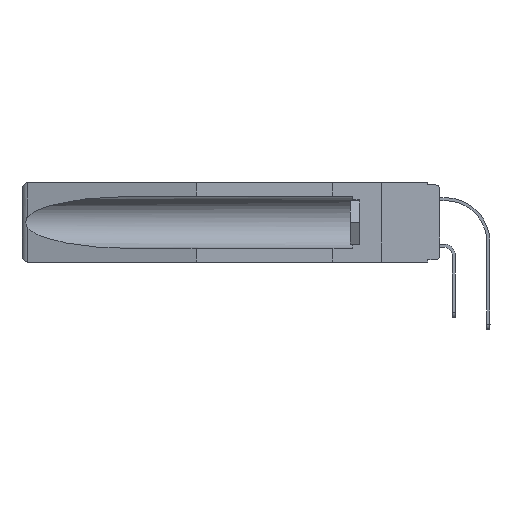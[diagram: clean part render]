
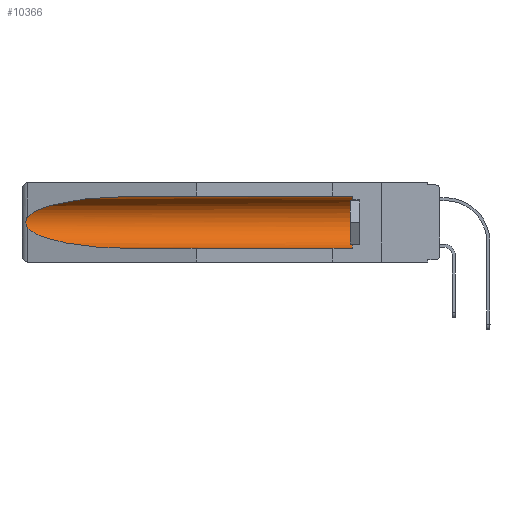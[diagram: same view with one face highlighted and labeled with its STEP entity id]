
A CAD part, left-side view. The second image highlights one B-rep face of the part: STEP entity #10366.
In plain terms, the highlighted cylindrical face has radius 2.857 mm (diameter 5.715 mm), a partial arc.
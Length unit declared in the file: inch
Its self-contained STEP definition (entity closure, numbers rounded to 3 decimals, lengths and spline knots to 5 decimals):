
#819 = VECTOR ( 'NONE', #11429, 39.37008 ) ;
#1091 = EDGE_CURVE ( 'NONE', #2972, #17838, #14023, .T. ) ;
#1241 = ORIENTED_EDGE ( 'NONE', *, *, #8715, .F. ) ;
#1884 = VECTOR ( 'NONE', #8492, 39.37008 ) ;
#2430 = CARTESIAN_POINT ( 'NONE',  ( 0.155, 1.07973, -0.284 ) ) ;
#2876 = CARTESIAN_POINT ( 'NONE',  ( 0.26597, 1.5296, -0.19026 ) ) ;
#2972 = VERTEX_POINT ( 'NONE', #4552 ) ;
#3889 = CYLINDRICAL_SURFACE ( 'NONE', #4646, 0.1125 ) ;
#4006 = CARTESIAN_POINT ( 'NONE',  ( 0.2675, 1.53308, -0.16763 ) ) ;
#4163 = CARTESIAN_POINT ( 'NONE',  ( 0.155, 1.07973, -0.059 ) ) ;
#4523 = EDGE_LOOP ( 'NONE', ( #17847, #11388, #7519, #1241, #16704, #6008 ) ) ;
#4552 = CARTESIAN_POINT ( 'NONE',  ( 0.155, 0.126, -0.059 ) ) ;
#4646 = AXIS2_PLACEMENT_3D ( 'NONE', #16730, #8152, #13783 ) ;
#4809 =( BOUNDED_CURVE ( )  B_SPLINE_CURVE ( 3, ( #4163, #5647, #17003, #9745 ),
 .UNSPECIFIED., .F., .F. ) 
 B_SPLINE_CURVE_WITH_KNOTS ( ( 4, 4 ),
 ( 4.71239, 6.08839 ),
 .UNSPECIFIED. ) 
 CURVE ( )  GEOMETRIC_REPRESENTATION_ITEM ( )  RATIONAL_B_SPLINE_CURVE ( ( 1., 0.848, 0.848, 1. ) ) 
 REPRESENTATION_ITEM ( '' )  );
#5072 = B_SPLINE_CURVE_WITH_KNOTS ( 'NONE', 3,
 ( #14075, #11043, #15450, #5665, #4006, #6882, #12518, #9936, #2876, #8532 ),
 .UNSPECIFIED., .F., .F.,
 ( 4, 2, 2, 2, 4 ),
 ( 0., 0.00029, 0.00058, 0.00087, 0.00117 ),
 .UNSPECIFIED. ) ;
#5316 = CARTESIAN_POINT ( 'NONE',  ( 0.26537, 1.52718, -0.14972 ) ) ;
#5380 = EDGE_CURVE ( 'NONE', #18029, #7241, #18037, .T. ) ;
#5389 = VERTEX_POINT ( 'NONE', #5316 ) ;
#5647 = CARTESIAN_POINT ( 'NONE',  ( 0.21114, 1.30732, -0.059 ) ) ;
#5665 = CARTESIAN_POINT ( 'NONE',  ( 0.2673, 1.5327, -0.16383 ) ) ;
#6008 = ORIENTED_EDGE ( 'NONE', *, *, #1091, .T. ) ;
#6882 = CARTESIAN_POINT ( 'NONE',  ( 0.2675, 1.53308, -0.17534 ) ) ;
#7241 = VERTEX_POINT ( 'NONE', #16741 ) ;
#7266 = EDGE_CURVE ( 'NONE', #17838, #5389, #4809, .T. ) ;
#7519 = ORIENTED_EDGE ( 'NONE', *, *, #5380, .T. ) ;
#8152 = DIRECTION ( 'NONE',  ( 0., 1., 0. ) ) ;
#8158 = CARTESIAN_POINT ( 'NONE',  ( 0.155, 1.07973, -0.059 ) ) ;
#8409 = CARTESIAN_POINT ( 'NONE',  ( 0.155, -0.30754, -0.284 ) ) ;
#8412 = EDGE_CURVE ( 'NONE', #5389, #18029, #5072, .T. ) ;
#8492 = DIRECTION ( 'NONE',  ( 0., 1., 0. ) ) ;
#8532 = CARTESIAN_POINT ( 'NONE',  ( 0.26537, 1.52718, -0.19328 ) ) ;
#8715 = EDGE_CURVE ( 'NONE', #15165, #7241, #18185, .T. ) ;
#9385 = CARTESIAN_POINT ( 'NONE',  ( 0.26537, 1.52718, -0.19328 ) ) ;
#9483 = CARTESIAN_POINT ( 'NONE',  ( 0.25451, 1.48313, -0.24835 ) ) ;
#9745 = CARTESIAN_POINT ( 'NONE',  ( 0.26537, 1.52718, -0.14972 ) ) ;
#9904 = AXIS2_PLACEMENT_3D ( 'NONE', #17911, #12299, #13489 ) ;
#9936 = CARTESIAN_POINT ( 'NONE',  ( 0.26655, 1.53094, -0.18657 ) ) ;
#10366 = ADVANCED_FACE ( 'NONE', ( #18115 ), #3889, .F. ) ;
#11043 = CARTESIAN_POINT ( 'NONE',  ( 0.26597, 1.52961, -0.15275 ) ) ;
#11251 = CARTESIAN_POINT ( 'NONE',  ( 0.155, -0.30754, -0.059 ) ) ;
#11282 = CARTESIAN_POINT ( 'NONE',  ( 0.26537, 1.52718, -0.19328 ) ) ;
#11388 = ORIENTED_EDGE ( 'NONE', *, *, #8412, .T. ) ;
#11429 = DIRECTION ( 'NONE',  ( 0., 1., 0. ) ) ;
#12299 = DIRECTION ( 'NONE',  ( 0., -1., 0. ) ) ;
#12518 = CARTESIAN_POINT ( 'NONE',  ( 0.2673, 1.53269, -0.17917 ) ) ;
#13031 = CARTESIAN_POINT ( 'NONE',  ( 0.155, 0.126, -0.284 ) ) ;
#13425 = CIRCLE ( 'NONE', #9904, 0.1125 ) ;
#13489 = DIRECTION ( 'NONE',  ( 0., 0., 1. ) ) ;
#13783 = DIRECTION ( 'NONE',  ( 0., 0., 1. ) ) ;
#14023 = LINE ( 'NONE', #11251, #819 ) ;
#14075 = CARTESIAN_POINT ( 'NONE',  ( 0.26537, 1.52718, -0.14972 ) ) ;
#15093 = CARTESIAN_POINT ( 'NONE',  ( 0.21114, 1.30732, -0.284 ) ) ;
#15165 = VERTEX_POINT ( 'NONE', #13031 ) ;
#15450 = CARTESIAN_POINT ( 'NONE',  ( 0.26654, 1.53092, -0.15636 ) ) ;
#16704 = ORIENTED_EDGE ( 'NONE', *, *, #18272, .T. ) ;
#16730 = CARTESIAN_POINT ( 'NONE',  ( 0.155, -0.30754, -0.1715 ) ) ;
#16741 = CARTESIAN_POINT ( 'NONE',  ( 0.155, 1.07973, -0.284 ) ) ;
#17003 = CARTESIAN_POINT ( 'NONE',  ( 0.25451, 1.48313, -0.09465 ) ) ;
#17838 = VERTEX_POINT ( 'NONE', #8158 ) ;
#17847 = ORIENTED_EDGE ( 'NONE', *, *, #7266, .T. ) ;
#17911 = CARTESIAN_POINT ( 'NONE',  ( 0.155, 0.126, -0.1715 ) ) ;
#18029 = VERTEX_POINT ( 'NONE', #11282 ) ;
#18037 =( BOUNDED_CURVE ( )  B_SPLINE_CURVE ( 3, ( #9385, #9483, #15093, #2430 ),
 .UNSPECIFIED., .F., .F. ) 
 B_SPLINE_CURVE_WITH_KNOTS ( ( 4, 4 ),
 ( 0.1948, 1.5708 ),
 .UNSPECIFIED. ) 
 CURVE ( )  GEOMETRIC_REPRESENTATION_ITEM ( )  RATIONAL_B_SPLINE_CURVE ( ( 1., 0.848, 0.848, 1. ) ) 
 REPRESENTATION_ITEM ( '' )  );
#18115 = FACE_OUTER_BOUND ( 'NONE', #4523, .T. ) ;
#18185 = LINE ( 'NONE', #8409, #1884 ) ;
#18272 = EDGE_CURVE ( 'NONE', #15165, #2972, #13425, .T. ) ;
